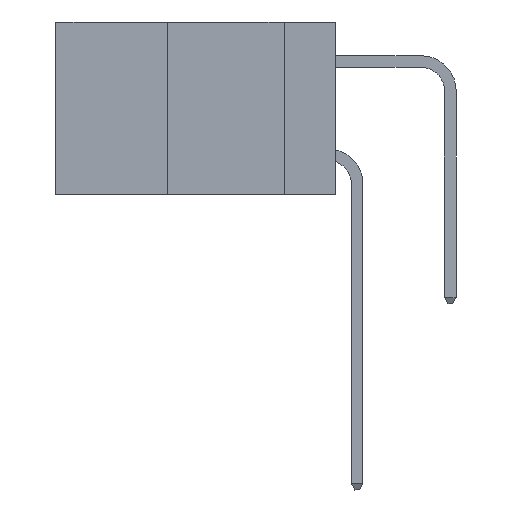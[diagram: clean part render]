
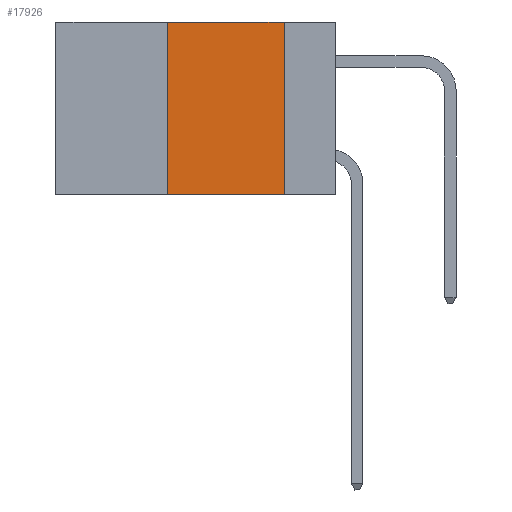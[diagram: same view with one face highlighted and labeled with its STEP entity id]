
A CAD part, left-side view. The second image highlights one B-rep face of the part: STEP entity #17926.
In plain terms, the highlighted planar face has unit normal (-1, 0, 0).
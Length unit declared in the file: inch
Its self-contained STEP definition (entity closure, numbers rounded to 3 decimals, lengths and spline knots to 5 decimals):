
#229 = DIRECTION ( 'NONE',  ( 0., 0., 1. ) ) ;
#385 = VERTEX_POINT ( 'NONE', #2383 ) ;
#1096 = CARTESIAN_POINT ( 'NONE',  ( 0., 0.11, 0. ) ) ;
#1440 = EDGE_CURVE ( 'NONE', #385, #7167, #5069, .T. ) ;
#1802 = AXIS2_PLACEMENT_3D ( 'NONE', #7131, #14357, #14438 ) ;
#1933 = ORIENTED_EDGE ( 'NONE', *, *, #3132, .F. ) ;
#2290 = EDGE_CURVE ( 'NONE', #5164, #385, #9999, .T. ) ;
#2360 = VECTOR ( 'NONE', #229, 39.37008 ) ;
#2383 = CARTESIAN_POINT ( 'NONE',  ( 0., 0.36, 0. ) ) ;
#3132 = EDGE_CURVE ( 'NONE', #7167, #14700, #7929, .T. ) ;
#3158 = DIRECTION ( 'NONE',  ( 0., -1., 0. ) ) ;
#3948 = CARTESIAN_POINT ( 'NONE',  ( 0., 0.36, 0. ) ) ;
#4195 = VECTOR ( 'NONE', #14957, 39.37008 ) ;
#4961 = ORIENTED_EDGE ( 'NONE', *, *, #17037, .T. ) ;
#5069 = LINE ( 'NONE', #15039, #4195 ) ;
#5164 = VERTEX_POINT ( 'NONE', #15883 ) ;
#6173 = VECTOR ( 'NONE', #8684, 39.37008 ) ;
#7131 = CARTESIAN_POINT ( 'NONE',  ( 0., 0.6, 0. ) ) ;
#7167 = VERTEX_POINT ( 'NONE', #14647 ) ;
#7929 = LINE ( 'NONE', #1096, #6173 ) ;
#8660 = FACE_OUTER_BOUND ( 'NONE', #23903, .T. ) ;
#8684 = DIRECTION ( 'NONE',  ( 0., 0., -1. ) ) ;
#9297 = ORIENTED_EDGE ( 'NONE', *, *, #2290, .F. ) ;
#9999 = LINE ( 'NONE', #3948, #2360 ) ;
#14357 = DIRECTION ( 'NONE',  ( 1., 0., 0. ) ) ;
#14396 = CARTESIAN_POINT ( 'NONE',  ( 0., 0.6, -0.37 ) ) ;
#14438 = DIRECTION ( 'NONE',  ( 0., 0., -1. ) ) ;
#14647 = CARTESIAN_POINT ( 'NONE',  ( 0., 0.11, 0. ) ) ;
#14700 = VERTEX_POINT ( 'NONE', #15855 ) ;
#14957 = DIRECTION ( 'NONE',  ( 0., -1., 0. ) ) ;
#15039 = CARTESIAN_POINT ( 'NONE',  ( 0., 0.6, 0. ) ) ;
#15855 = CARTESIAN_POINT ( 'NONE',  ( 0., 0.11, -0.37 ) ) ;
#15883 = CARTESIAN_POINT ( 'NONE',  ( 0., 0.36, -0.37 ) ) ;
#17037 = EDGE_CURVE ( 'NONE', #5164, #14700, #17133, .T. ) ;
#17133 = LINE ( 'NONE', #14396, #24197 ) ;
#17926 = ADVANCED_FACE ( 'NONE', ( #8660 ), #18484, .F. ) ;
#18484 = PLANE ( 'NONE',  #1802 ) ;
#23903 = EDGE_LOOP ( 'NONE', ( #1933, #24337, #9297, #4961 ) ) ;
#24197 = VECTOR ( 'NONE', #3158, 39.37008 ) ;
#24337 = ORIENTED_EDGE ( 'NONE', *, *, #1440, .F. ) ;
